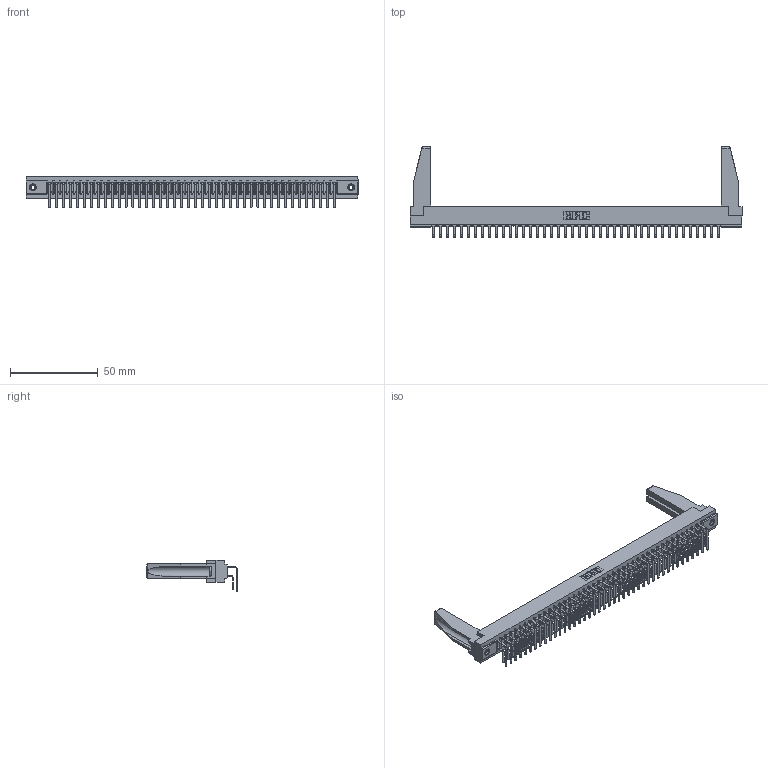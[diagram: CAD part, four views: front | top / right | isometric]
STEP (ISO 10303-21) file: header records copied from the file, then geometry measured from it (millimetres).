
FILE_DESCRIPTION (( 'STEP AP203' ), '1' );
FILE_NAME ('307-042-459-178.STEP', '2020-09-29T17:38:55', ( '' ), ( '' ), 'SwSTEP 2.0', 'SolidWorks 2020', '' );
FILE_SCHEMA (( 'CONFIG_CONTROL_DESIGN' ));
Length unit declared in the file: inch
Products named in the file (6): 307-042-459-178; 307-220-078; 307 Part_.156 Dia Mounting Holes; 307-290-001_558 559 - 1 (Single); 345-250-001_345-250-001-102; 307-290-001_559 - 2 (Single)
Assembly tree (89 placements, depth 2):
  307-042-459-178
    307 Part_.156 Dia Mounting Holes
    307-290-001_558 559 - 1 (Single)  x42
    307-290-001_559 - 2 (Single)  x42
    307-220-078  x2
    345-250-001_345-250-001-102  x2
Bounding box: 189.43 x 51.4 x 18.07 mm (x, y, z)
Volume: 24509.7 mm3; surface area: 31098.9 mm2
Topology: 89 solids, 89 shells, 4491 faces, 12581 edges, 8150 vertices
Faces by surface type: plane 2926, cylinder 1463, sphere 86, cone 12, torus 4
Entity records: 41236 total; most frequent: CARTESIAN_POINT 6758, ORIENTED_EDGE 6656, DIRECTION 6572, EDGE_CURVE 3328, LINE 2556, VECTOR 2556, VERTEX_POINT 2152, AXIS2_PLACEMENT_3D 2008
